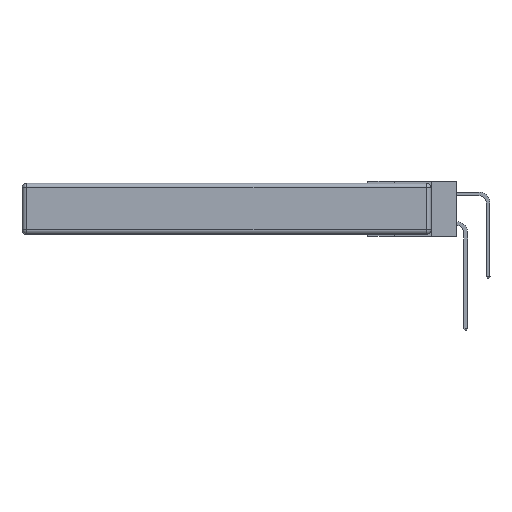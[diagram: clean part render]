
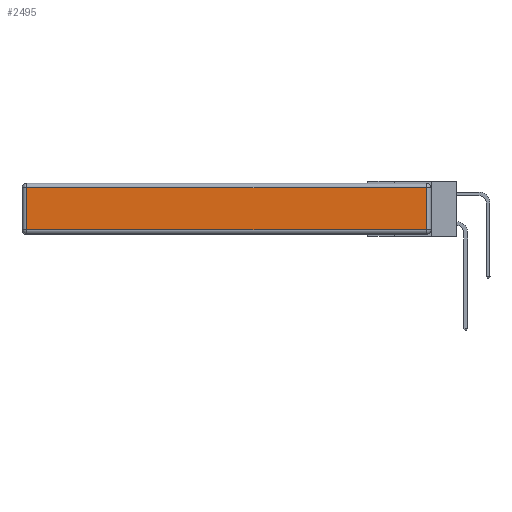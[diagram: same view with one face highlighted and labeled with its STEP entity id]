
A CAD part, left-side view. The second image highlights one B-rep face of the part: STEP entity #2495.
In plain terms, the highlighted planar face has unit normal (-1, 0, 0).
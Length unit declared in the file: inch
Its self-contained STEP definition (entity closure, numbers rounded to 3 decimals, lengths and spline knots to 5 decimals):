
#157 = EDGE_CURVE ( 'NONE', #6676, #5145, #6750, .T. ) ;
#191 = ORIENTED_EDGE ( 'NONE', *, *, #13705, .T. ) ;
#606 = DIRECTION ( 'NONE',  ( 0., -1., 0. ) ) ;
#1584 = CARTESIAN_POINT ( 'NONE',  ( 0., 2.72, -0.03 ) ) ;
#1911 = LINE ( 'NONE', #12241, #7337 ) ;
#2153 = LINE ( 'NONE', #13409, #11305 ) ;
#2352 = VECTOR ( 'NONE', #606, 39.37008 ) ;
#2493 = PLANE ( 'NONE',  #13755 ) ;
#2495 = ADVANCED_FACE ( 'NONE', ( #11345 ), #2493, .T. ) ;
#3314 = EDGE_LOOP ( 'NONE', ( #191, #13911, #7192, #4897 ) ) ;
#4873 = VECTOR ( 'NONE', #9524, 39.37008 ) ;
#4897 = ORIENTED_EDGE ( 'NONE', *, *, #157, .T. ) ;
#5145 = VERTEX_POINT ( 'NONE', #5641 ) ;
#5393 = EDGE_CURVE ( 'NONE', #8697, #6676, #1911, .T. ) ;
#5491 = VERTEX_POINT ( 'NONE', #7296 ) ;
#5641 = CARTESIAN_POINT ( 'NONE',  ( 0., 2.72, -0.313 ) ) ;
#6676 = VERTEX_POINT ( 'NONE', #1584 ) ;
#6750 = LINE ( 'NONE', #12873, #4873 ) ;
#7192 = ORIENTED_EDGE ( 'NONE', *, *, #5393, .T. ) ;
#7296 = CARTESIAN_POINT ( 'NONE',  ( 0., 0.03, -0.313 ) ) ;
#7337 = VECTOR ( 'NONE', #10265, 39.37008 ) ;
#8064 = CARTESIAN_POINT ( 'NONE',  ( 0., 0., -0.343 ) ) ;
#8251 = EDGE_CURVE ( 'NONE', #5491, #8697, #2153, .T. ) ;
#8463 = LINE ( 'NONE', #10422, #2352 ) ;
#8697 = VERTEX_POINT ( 'NONE', #13859 ) ;
#9160 = DIRECTION ( 'NONE',  ( 0., 0., 1. ) ) ;
#9524 = DIRECTION ( 'NONE',  ( 0., 0., -1. ) ) ;
#10247 = DIRECTION ( 'NONE',  ( -1., 0., 0. ) ) ;
#10265 = DIRECTION ( 'NONE',  ( 0., 1., 0. ) ) ;
#10422 = CARTESIAN_POINT ( 'NONE',  ( 0., 0., -0.313 ) ) ;
#11305 = VECTOR ( 'NONE', #12654, 39.37008 ) ;
#11345 = FACE_OUTER_BOUND ( 'NONE', #3314, .T. ) ;
#12241 = CARTESIAN_POINT ( 'NONE',  ( 0., 2.75, -0.03 ) ) ;
#12654 = DIRECTION ( 'NONE',  ( 0., 0., 1. ) ) ;
#12873 = CARTESIAN_POINT ( 'NONE',  ( 0., 2.72, -0.343 ) ) ;
#13409 = CARTESIAN_POINT ( 'NONE',  ( 0., 0.03, -0.343 ) ) ;
#13705 = EDGE_CURVE ( 'NONE', #5145, #5491, #8463, .T. ) ;
#13755 = AXIS2_PLACEMENT_3D ( 'NONE', #8064, #10247, #9160 ) ;
#13859 = CARTESIAN_POINT ( 'NONE',  ( 0., 0.03, -0.03 ) ) ;
#13911 = ORIENTED_EDGE ( 'NONE', *, *, #8251, .T. ) ;
